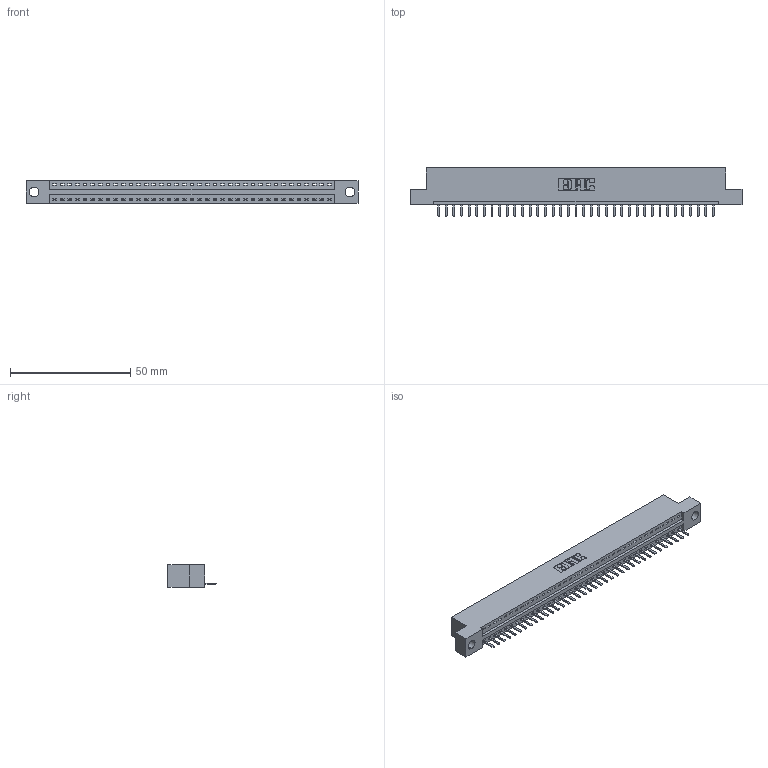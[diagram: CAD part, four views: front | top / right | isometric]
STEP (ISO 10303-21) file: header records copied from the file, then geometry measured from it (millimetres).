
FILE_DESCRIPTION (( 'STEP AP203' ), '1' );
FILE_NAME ('396-037-520-104.STEP', '2019-10-27T17:22:34', ( '' ), ( '' ), 'SwSTEP 2.0', 'SolidWorks 2016', '' );
FILE_SCHEMA (( 'CONFIG_CONTROL_DESIGN' ));
Length unit declared in the file: inch
Products named in the file (3): 346 Part_Flush Mounting Lugs - 0.156 Dia-TH; 396-037-520-104; 345-292-001_345-293-120
Assembly tree (38 placements, depth 2):
  396-037-520-104
    346 Part_Flush Mounting Lugs - 0.156 Dia-TH
    345-292-001_345-293-120  x37
Bounding box: 138.05 x 20.02 x 9.4 mm (x, y, z)
Volume: 12985.6 mm3; surface area: 15626.1 mm2
Topology: 38 solids, 38 shells, 2416 faces, 7137 edges, 4658 vertices
Faces by surface type: plane 1630, cylinder 786
Entity records: 23753 total; most frequent: CARTESIAN_POINT 4091, ORIENTED_EDGE 4050, DIRECTION 3603, EDGE_CURVE 2025, LINE 1741, VECTOR 1741, VERTEX_POINT 1346, AXIS2_PLACEMENT_3D 931
